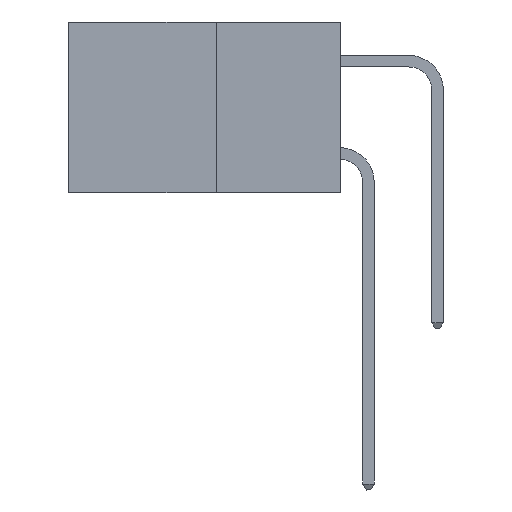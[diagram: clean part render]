
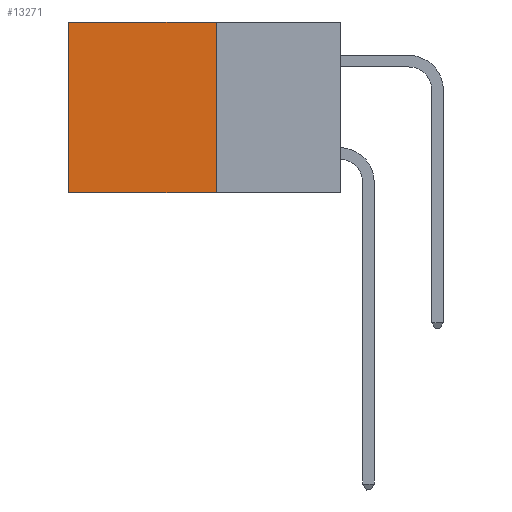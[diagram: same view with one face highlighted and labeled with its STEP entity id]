
A CAD part, left-side view. The second image highlights one B-rep face of the part: STEP entity #13271.
In plain terms, the highlighted planar face has unit normal (-1, 0, 0).
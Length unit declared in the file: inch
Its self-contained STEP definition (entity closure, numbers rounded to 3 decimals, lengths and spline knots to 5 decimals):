
#1179 = CARTESIAN_POINT ( 'NONE',  ( 0.277, 0.27, -0.37 ) ) ;
#1947 = CARTESIAN_POINT ( 'NONE',  ( 0.277, 0.27, -0.37 ) ) ;
#2207 = LINE ( 'NONE', #14858, #5254 ) ;
#2639 = VECTOR ( 'NONE', #15515, 39.37008 ) ;
#3319 = DIRECTION ( 'NONE',  ( 0., 0., -1. ) ) ;
#4110 = CARTESIAN_POINT ( 'NONE',  ( 0.277, 0.59, 0. ) ) ;
#4840 = EDGE_CURVE ( 'NONE', #15979, #9300, #12786, .T. ) ;
#4854 = AXIS2_PLACEMENT_3D ( 'NONE', #1947, #5843, #14673 ) ;
#5254 = VECTOR ( 'NONE', #8592, 39.37008 ) ;
#5790 = FACE_OUTER_BOUND ( 'NONE', #9285, .T. ) ;
#5843 = DIRECTION ( 'NONE',  ( 1., 0., 0. ) ) ;
#6568 = EDGE_CURVE ( 'NONE', #15741, #15979, #8631, .T. ) ;
#7317 = CARTESIAN_POINT ( 'NONE',  ( 0.277, 0.59, -0.37 ) ) ;
#7747 = ORIENTED_EDGE ( 'NONE', *, *, #4840, .F. ) ;
#7755 = ORIENTED_EDGE ( 'NONE', *, *, #9708, .T. ) ;
#8085 = VERTEX_POINT ( 'NONE', #4110 ) ;
#8250 = VECTOR ( 'NONE', #15122, 39.37008 ) ;
#8592 = DIRECTION ( 'NONE',  ( 0., 1., 0. ) ) ;
#8631 = LINE ( 'NONE', #8850, #8250 ) ;
#8850 = CARTESIAN_POINT ( 'NONE',  ( 0.277, 0.27, -0.37 ) ) ;
#9285 = EDGE_LOOP ( 'NONE', ( #10442, #7747, #9892, #7755 ) ) ;
#9300 = VERTEX_POINT ( 'NONE', #7317 ) ;
#9682 = CARTESIAN_POINT ( 'NONE',  ( 0.277, 0.59, -0.37 ) ) ;
#9708 = EDGE_CURVE ( 'NONE', #15741, #8085, #2207, .T. ) ;
#9892 = ORIENTED_EDGE ( 'NONE', *, *, #6568, .F. ) ;
#10442 = ORIENTED_EDGE ( 'NONE', *, *, #11230, .T. ) ;
#11230 = EDGE_CURVE ( 'NONE', #8085, #9300, #13960, .T. ) ;
#12786 = LINE ( 'NONE', #14247, #2639 ) ;
#13163 = VECTOR ( 'NONE', #3319, 39.37008 ) ;
#13271 = ADVANCED_FACE ( 'NONE', ( #5790 ), #13410, .F. ) ;
#13410 = PLANE ( 'NONE',  #4854 ) ;
#13448 = CARTESIAN_POINT ( 'NONE',  ( 0.277, 0.27, 0. ) ) ;
#13960 = LINE ( 'NONE', #9682, #13163 ) ;
#14247 = CARTESIAN_POINT ( 'NONE',  ( 0.277, 0.27, -0.37 ) ) ;
#14673 = DIRECTION ( 'NONE',  ( 0., 0., -1. ) ) ;
#14858 = CARTESIAN_POINT ( 'NONE',  ( 0.277, 0.27, 0. ) ) ;
#15122 = DIRECTION ( 'NONE',  ( 0., 0., -1. ) ) ;
#15515 = DIRECTION ( 'NONE',  ( 0., 1., 0. ) ) ;
#15741 = VERTEX_POINT ( 'NONE', #13448 ) ;
#15979 = VERTEX_POINT ( 'NONE', #1179 ) ;
